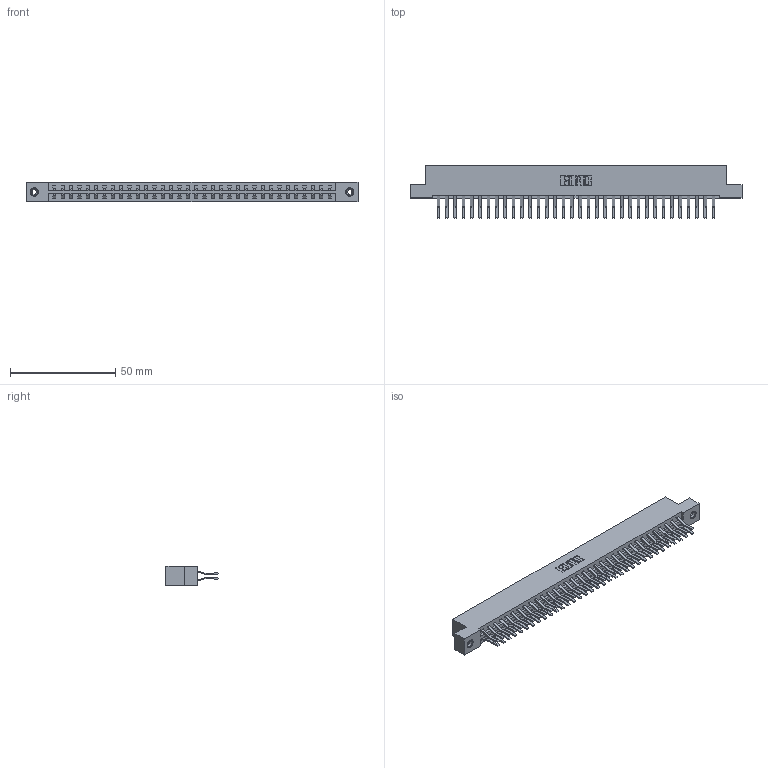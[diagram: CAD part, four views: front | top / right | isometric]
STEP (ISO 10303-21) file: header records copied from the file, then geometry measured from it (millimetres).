
FILE_DESCRIPTION (( 'STEP AP203' ), '1' );
FILE_NAME ('387-068-560-208.STEP', '2019-10-19T22:21:33', ( '' ), ( '' ), 'SwSTEP 2.0', 'SolidWorks 2016', '' );
FILE_SCHEMA (( 'CONFIG_CONTROL_DESIGN' ));
Length unit declared in the file: inch
Products named in the file (4): 345-250-001_345-250-003-102; 387-068-560-208; 345-292-001_560 Tail; 337 Part_Flush Mounting Lugs - 0.156 Dia-TI
Assembly tree (71 placements, depth 2):
  387-068-560-208
    337 Part_Flush Mounting Lugs - 0.156 Dia-TI
    345-292-001_560 Tail  x68
    345-250-001_345-250-003-102  x2
Bounding box: 157.73 x 24.78 x 9.4 mm (x, y, z)
Volume: 16956 mm3; surface area: 20405 mm2
Topology: 71 solids, 71 shells, 3982 faces, 11803 edges, 7770 vertices
Faces by surface type: plane 2686, cylinder 1280, cone 12, torus 4
Entity records: 28670 total; most frequent: CARTESIAN_POINT 4817, ORIENTED_EDGE 4746, DIRECTION 4147, EDGE_CURVE 2373, VECTOR 2221, LINE 2221, VERTEX_POINT 1576, AXIS2_PLACEMENT_3D 963
